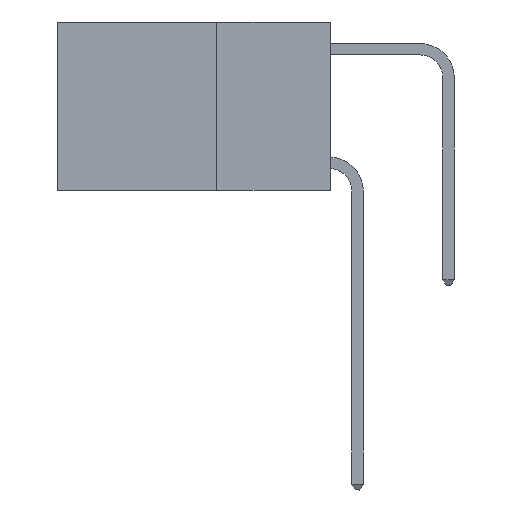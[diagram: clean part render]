
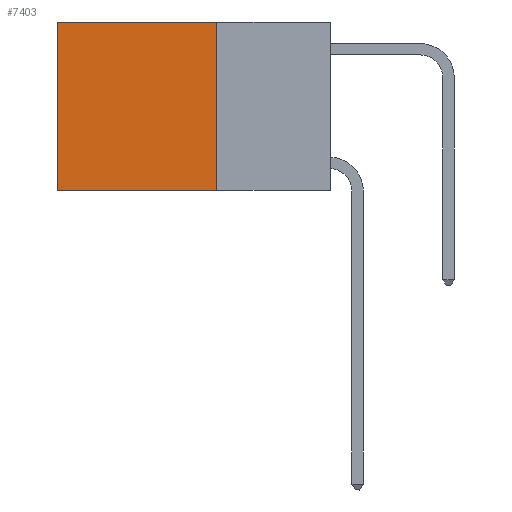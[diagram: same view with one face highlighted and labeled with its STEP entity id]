
A CAD part, left-side view. The second image highlights one B-rep face of the part: STEP entity #7403.
In plain terms, the highlighted planar face has unit normal (-1, 0, 0).
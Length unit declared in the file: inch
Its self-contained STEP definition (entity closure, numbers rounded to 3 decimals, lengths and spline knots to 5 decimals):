
#1453 = EDGE_CURVE ( 'NONE', #3373, #2966, #4707, .T. ) ;
#1455 = CARTESIAN_POINT ( 'NONE',  ( 0.2625, 0.6, 0. ) ) ;
#2103 = ORIENTED_EDGE ( 'NONE', *, *, #4976, .F. ) ;
#2489 = VECTOR ( 'NONE', #17121, 39.37008 ) ;
#2516 = VECTOR ( 'NONE', #17131, 39.37008 ) ;
#2840 = EDGE_CURVE ( 'NONE', #15511, #17414, #10238, .T. ) ;
#2966 = VERTEX_POINT ( 'NONE', #18096 ) ;
#3373 = VERTEX_POINT ( 'NONE', #14872 ) ;
#3730 = CARTESIAN_POINT ( 'NONE',  ( 0.2625, 0.25, 0. ) ) ;
#4707 = LINE ( 'NONE', #14293, #2489 ) ;
#4976 = EDGE_CURVE ( 'NONE', #15511, #3373, #7467, .T. ) ;
#5350 = AXIS2_PLACEMENT_3D ( 'NONE', #6170, #9492, #6550 ) ;
#6170 = CARTESIAN_POINT ( 'NONE',  ( 0.2625, 0.25, 0. ) ) ;
#6324 = LINE ( 'NONE', #1455, #2516 ) ;
#6550 = DIRECTION ( 'NONE',  ( 0., 0., -1. ) ) ;
#6636 = ORIENTED_EDGE ( 'NONE', *, *, #1453, .F. ) ;
#7071 = EDGE_LOOP ( 'NONE', ( #7530, #6636, #2103, #17983 ) ) ;
#7403 = ADVANCED_FACE ( 'NONE', ( #10527 ), #12099, .F. ) ;
#7467 = LINE ( 'NONE', #3730, #16513 ) ;
#7530 = ORIENTED_EDGE ( 'NONE', *, *, #13999, .T. ) ;
#7637 = DIRECTION ( 'NONE',  ( 0., 0., -1. ) ) ;
#9492 = DIRECTION ( 'NONE',  ( 1., 0., 0. ) ) ;
#10238 = LINE ( 'NONE', #10855, #12866 ) ;
#10527 = FACE_OUTER_BOUND ( 'NONE', #7071, .T. ) ;
#10855 = CARTESIAN_POINT ( 'NONE',  ( 0.2625, 0.25, 0. ) ) ;
#12099 = PLANE ( 'NONE',  #5350 ) ;
#12866 = VECTOR ( 'NONE', #15338, 39.37008 ) ;
#13999 = EDGE_CURVE ( 'NONE', #17414, #2966, #6324, .T. ) ;
#14293 = CARTESIAN_POINT ( 'NONE',  ( 0.2625, 0.25, -0.37 ) ) ;
#14872 = CARTESIAN_POINT ( 'NONE',  ( 0.2625, 0.25, -0.37 ) ) ;
#15338 = DIRECTION ( 'NONE',  ( 0., 1., 0. ) ) ;
#15511 = VERTEX_POINT ( 'NONE', #16401 ) ;
#16401 = CARTESIAN_POINT ( 'NONE',  ( 0.2625, 0.25, 0. ) ) ;
#16513 = VECTOR ( 'NONE', #7637, 39.37008 ) ;
#16866 = CARTESIAN_POINT ( 'NONE',  ( 0.2625, 0.6, 0. ) ) ;
#17121 = DIRECTION ( 'NONE',  ( 0., 1., 0. ) ) ;
#17131 = DIRECTION ( 'NONE',  ( 0., 0., -1. ) ) ;
#17414 = VERTEX_POINT ( 'NONE', #16866 ) ;
#17983 = ORIENTED_EDGE ( 'NONE', *, *, #2840, .T. ) ;
#18096 = CARTESIAN_POINT ( 'NONE',  ( 0.2625, 0.6, -0.37 ) ) ;
